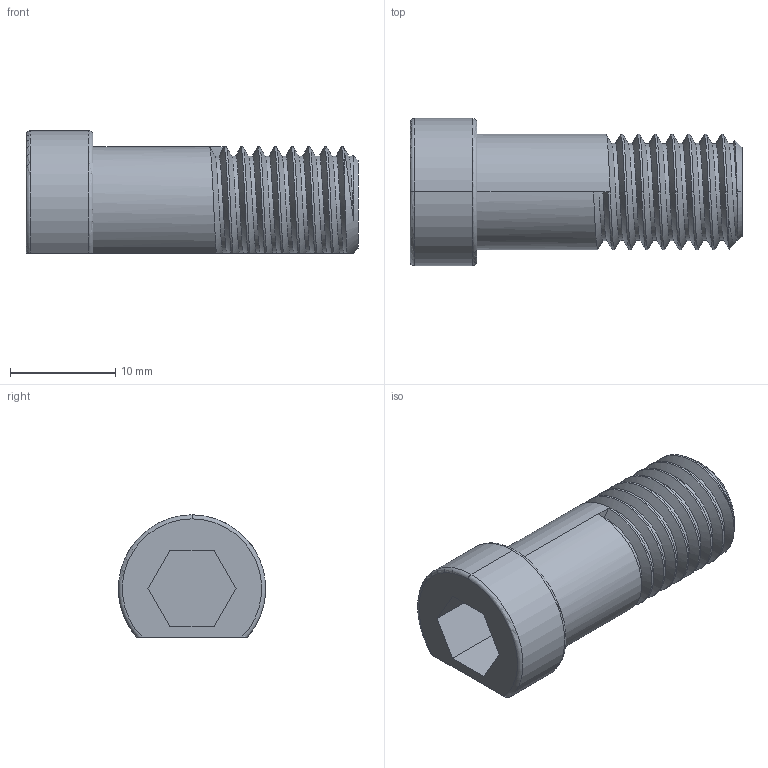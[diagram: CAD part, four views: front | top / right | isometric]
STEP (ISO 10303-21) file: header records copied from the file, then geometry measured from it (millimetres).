
FILE_DESCRIPTION (( 'STEP AP203' ), '1' );
FILE_NAME ('AF-HF-LR-PRT-003-STEP.STEP', '2020-11-01T01:30:28', ( '' ), ( '' ), 'SwSTEP 2.0', 'SolidWorks 2018', '' );
FILE_SCHEMA (( 'CONFIG_CONTROL_DESIGN' ));
Length unit declared in the file: inch
Products named in the file (1): AF-HF-LR-PRT-003-STEP
Bounding box: 31.5 x 13.95 x 11.6 mm (x, y, z)
Volume: 2452.9 mm3; surface area: 1818.1 mm2
Topology: 1 solids, 1 shells, 69 faces, 181 edges, 115 vertices
Faces by surface type: plane 42, cylinder 19, torus 3, bspline 3, cone 2
Entity records: 3629 total; most frequent: CARTESIAN_POINT 2012, ORIENTED_EDGE 362, DIRECTION 267, EDGE_CURVE 181, VERTEX_POINT 115, LINE 107, VECTOR 107, AXIS2_PLACEMENT_3D 80
